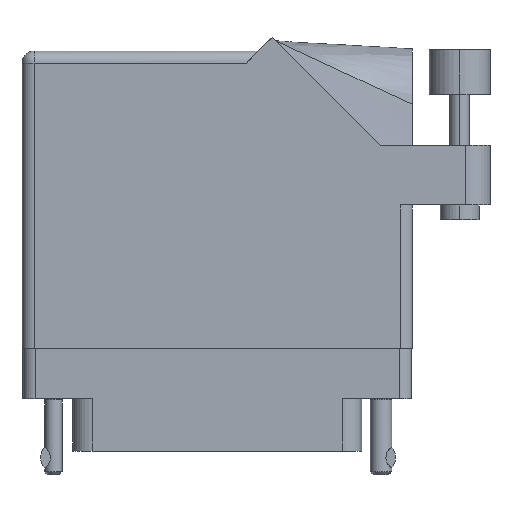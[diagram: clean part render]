
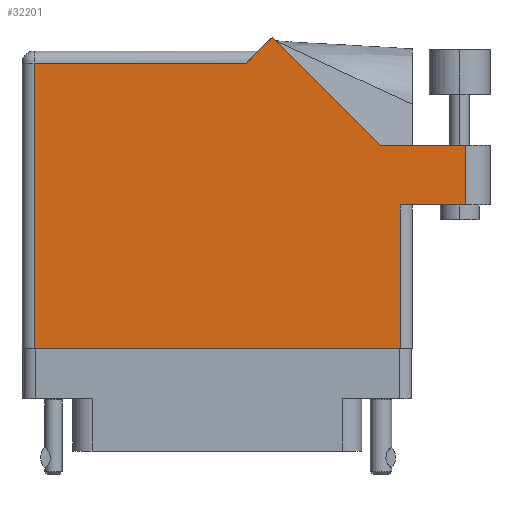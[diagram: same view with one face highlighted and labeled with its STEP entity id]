
A CAD part, front view. The second image highlights one B-rep face of the part: STEP entity #32201.
In plain terms, the highlighted face is planar.
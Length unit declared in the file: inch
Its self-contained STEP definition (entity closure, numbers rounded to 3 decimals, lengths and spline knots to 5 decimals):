
#414 = VERTEX_POINT ( 'NONE', #5378 ) ;
#433 = VERTEX_POINT ( 'NONE', #19252 ) ;
#1618 = CARTESIAN_POINT ( 'NONE',  ( 0.062, 0., 0. ) ) ;
#1822 = LINE ( 'NONE', #21179, #16264 ) ;
#3325 = LINE ( 'NONE', #37926, #31690 ) ;
#3778 = CARTESIAN_POINT ( 'NONE',  ( 1.155, 1.468, 0. ) ) ;
#4206 = EDGE_LOOP ( 'NONE', ( #29491, #37325, #22051, #36603, #34757, #31533, #31971, #23642, #41828 ) ) ;
#5141 = VECTOR ( 'NONE', #32708, 39.37008 ) ;
#5378 = CARTESIAN_POINT ( 'NONE',  ( 2.285, 0.737, 0. ) ) ;
#6459 = CARTESIAN_POINT ( 'NONE',  ( 1.948, 0., 0. ) ) ;
#7014 = DIRECTION ( 'NONE',  ( 0., 1., 0. ) ) ;
#7061 = LINE ( 'NONE', #23953, #40798 ) ;
#7718 = VECTOR ( 'NONE', #34351, 39.37008 ) ;
#7849 = DIRECTION ( 'NONE',  ( -1., 0., 0. ) ) ;
#7876 = CARTESIAN_POINT ( 'NONE',  ( 2.41, 1.044, 0. ) ) ;
#10361 = LINE ( 'NONE', #32082, #18901 ) ;
#11125 = DIRECTION ( 'NONE',  ( -1., 0., 0. ) ) ;
#11413 = LINE ( 'NONE', #17328, #14039 ) ;
#12965 = VERTEX_POINT ( 'NONE', #1618 ) ;
#13589 = FACE_OUTER_BOUND ( 'NONE', #4206, .T. ) ;
#14039 = VECTOR ( 'NONE', #7014, 39.37008 ) ;
#14518 = DIRECTION ( 'NONE',  ( 0., 0., -1. ) ) ;
#14636 = VECTOR ( 'NONE', #27312, 39.37008 ) ;
#15974 = EDGE_CURVE ( 'NONE', #414, #17860, #25935, .T. ) ;
#16264 = VECTOR ( 'NONE', #27666, 39.37008 ) ;
#16451 = EDGE_CURVE ( 'NONE', #38603, #414, #23742, .T. ) ;
#16760 = EDGE_CURVE ( 'NONE', #21702, #433, #10361, .T. ) ;
#17083 = DIRECTION ( 'NONE',  ( 1., 0., 0. ) ) ;
#17328 = CARTESIAN_POINT ( 'NONE',  ( 1.948, 0.737, 0. ) ) ;
#17860 = VERTEX_POINT ( 'NONE', #18193 ) ;
#18193 = CARTESIAN_POINT ( 'NONE',  ( 2.285, 1.044, 0. ) ) ;
#18901 = VECTOR ( 'NONE', #7849, 39.37008 ) ;
#19007 = EDGE_CURVE ( 'NONE', #433, #12965, #42033, .T. ) ;
#19252 = CARTESIAN_POINT ( 'NONE',  ( 0.062, 1.468, 0. ) ) ;
#19323 = AXIS2_PLACEMENT_3D ( 'NONE', #31304, #14518, #11125 ) ;
#20175 = CARTESIAN_POINT ( 'NONE',  ( 1.948, 0.737, 0. ) ) ;
#21179 = CARTESIAN_POINT ( 'NONE',  ( 1.84442, 1.044, 0. ) ) ;
#21702 = VERTEX_POINT ( 'NONE', #3778 ) ;
#21768 = EDGE_CURVE ( 'NONE', #12965, #27092, #7061, .T. ) ;
#22051 = ORIENTED_EDGE ( 'NONE', *, *, #23630, .T. ) ;
#23416 = CARTESIAN_POINT ( 'NONE',  ( 2.285, 1.044, 0. ) ) ;
#23539 = CARTESIAN_POINT ( 'NONE',  ( 2.01, 0.737, 0. ) ) ;
#23630 = EDGE_CURVE ( 'NONE', #17860, #24642, #39565, .T. ) ;
#23642 = ORIENTED_EDGE ( 'NONE', *, *, #21768, .T. ) ;
#23742 = LINE ( 'NONE', #23539, #14636 ) ;
#23953 = CARTESIAN_POINT ( 'NONE',  ( 0., 0., 0. ) ) ;
#24642 = VERTEX_POINT ( 'NONE', #44251 ) ;
#25488 = VERTEX_POINT ( 'NONE', #33282 ) ;
#25536 = CARTESIAN_POINT ( 'NONE',  ( 0.062, 0., 0. ) ) ;
#25935 = LINE ( 'NONE', #23416, #7718 ) ;
#26738 = VECTOR ( 'NONE', #35076, 39.37008 ) ;
#27092 = VERTEX_POINT ( 'NONE', #6459 ) ;
#27312 = DIRECTION ( 'NONE',  ( 1., 0., 0. ) ) ;
#27666 = DIRECTION ( 'NONE',  ( -0.707, 0.707, 0. ) ) ;
#29491 = ORIENTED_EDGE ( 'NONE', *, *, #16451, .T. ) ;
#31304 = CARTESIAN_POINT ( 'NONE',  ( 0., 1.53, 0. ) ) ;
#31533 = ORIENTED_EDGE ( 'NONE', *, *, #16760, .T. ) ;
#31690 = VECTOR ( 'NONE', #41369, 39.37008 ) ;
#31971 = ORIENTED_EDGE ( 'NONE', *, *, #19007, .T. ) ;
#32082 = CARTESIAN_POINT ( 'NONE',  ( 0., 1.468, 0. ) ) ;
#32201 = ADVANCED_FACE ( 'NONE', ( #13589 ), #34727, .F. ) ;
#32708 = DIRECTION ( 'NONE',  ( 0., -1., 0. ) ) ;
#33282 = CARTESIAN_POINT ( 'NONE',  ( 1.28771, 1.60071, 0. ) ) ;
#34351 = DIRECTION ( 'NONE',  ( 0., 1., 0. ) ) ;
#34727 = PLANE ( 'NONE',  #19323 ) ;
#34757 = ORIENTED_EDGE ( 'NONE', *, *, #40130, .T. ) ;
#35076 = DIRECTION ( 'NONE',  ( -1., 0., 0. ) ) ;
#36603 = ORIENTED_EDGE ( 'NONE', *, *, #38978, .T. ) ;
#37325 = ORIENTED_EDGE ( 'NONE', *, *, #15974, .T. ) ;
#37926 = CARTESIAN_POINT ( 'NONE',  ( 1.217, 1.53, 0. ) ) ;
#38603 = VERTEX_POINT ( 'NONE', #20175 ) ;
#38978 = EDGE_CURVE ( 'NONE', #24642, #25488, #1822, .T. ) ;
#39565 = LINE ( 'NONE', #7876, #26738 ) ;
#40130 = EDGE_CURVE ( 'NONE', #25488, #21702, #3325, .T. ) ;
#40798 = VECTOR ( 'NONE', #17083, 39.37008 ) ;
#41369 = DIRECTION ( 'NONE',  ( -0.707, -0.707, 0. ) ) ;
#41828 = ORIENTED_EDGE ( 'NONE', *, *, #42221, .T. ) ;
#42033 = LINE ( 'NONE', #25536, #5141 ) ;
#42221 = EDGE_CURVE ( 'NONE', #27092, #38603, #11413, .T. ) ;
#44251 = CARTESIAN_POINT ( 'NONE',  ( 1.84442, 1.044, 0. ) ) ;
